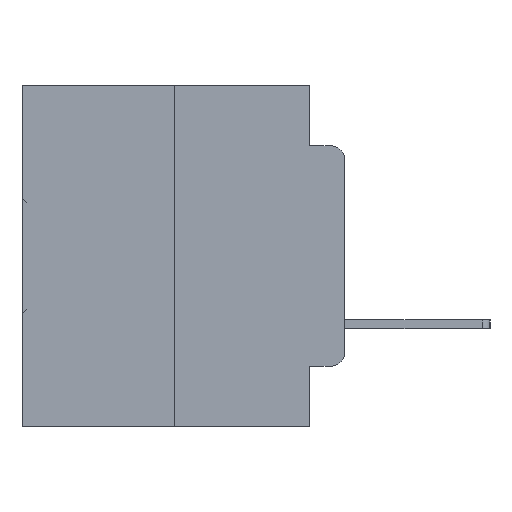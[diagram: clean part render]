
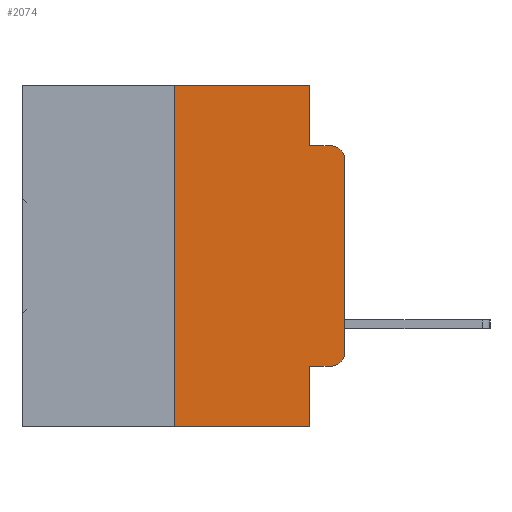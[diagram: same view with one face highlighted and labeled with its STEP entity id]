
A CAD part, left-side view. The second image highlights one B-rep face of the part: STEP entity #2074.
In plain terms, the highlighted planar face has unit normal (-1, 0, 0).
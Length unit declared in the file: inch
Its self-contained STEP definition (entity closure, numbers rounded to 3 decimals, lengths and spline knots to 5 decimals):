
#961 = EDGE_CURVE ( 'NONE', #13620, #11666, #12895, .T. ) ;
#1008 = VECTOR ( 'NONE', #7044, 39.37008 ) ;
#1554 = DIRECTION ( 'NONE',  ( 0., -1., 0. ) ) ;
#2074 = ADVANCED_FACE ( 'NONE', ( #23694 ), #25419, .F. ) ;
#2277 = ORIENTED_EDGE ( 'NONE', *, *, #2751, .T. ) ;
#2463 = ORIENTED_EDGE ( 'NONE', *, *, #961, .T. ) ;
#2751 = EDGE_CURVE ( 'NONE', #11666, #20165, #25672, .T. ) ;
#3891 = CARTESIAN_POINT ( 'NONE',  ( 0., 0.473, -0.5 ) ) ;
#4189 = ORIENTED_EDGE ( 'NONE', *, *, #15668, .F. ) ;
#5625 = LINE ( 'NONE', #25116, #13402 ) ;
#6487 = VERTEX_POINT ( 'NONE', #28314 ) ;
#6634 = LINE ( 'NONE', #17175, #19680 ) ;
#6671 = CARTESIAN_POINT ( 'NONE',  ( 0., 0.25, 0. ) ) ;
#6856 = EDGE_CURVE ( 'NONE', #26760, #13575, #19424, .T. ) ;
#7044 = DIRECTION ( 'NONE',  ( 0., 0., 1. ) ) ;
#7055 = DIRECTION ( 'NONE',  ( 0., 0., -1. ) ) ;
#7791 = ORIENTED_EDGE ( 'NONE', *, *, #6856, .T. ) ;
#8467 = CARTESIAN_POINT ( 'NONE',  ( 0., 0.051, -0.0885 ) ) ;
#8584 = ORIENTED_EDGE ( 'NONE', *, *, #30925, .F. ) ;
#8736 = AXIS2_PLACEMENT_3D ( 'NONE', #24629, #9180, #27189 ) ;
#8743 = LINE ( 'NONE', #14873, #1008 ) ;
#8964 = CARTESIAN_POINT ( 'NONE',  ( 0., 0.051, -0.4115 ) ) ;
#9180 = DIRECTION ( 'NONE',  ( -1., 0., 0. ) ) ;
#9181 = ORIENTED_EDGE ( 'NONE', *, *, #14524, .T. ) ;
#9754 = ORIENTED_EDGE ( 'NONE', *, *, #27592, .F. ) ;
#10502 = ORIENTED_EDGE ( 'NONE', *, *, #16811, .F. ) ;
#10653 = ORIENTED_EDGE ( 'NONE', *, *, #20800, .F. ) ;
#10763 = VERTEX_POINT ( 'NONE', #29283 ) ;
#11415 = CARTESIAN_POINT ( 'NONE',  ( 0., 0.25, -0.5 ) ) ;
#11505 = CARTESIAN_POINT ( 'NONE',  ( 0., 0.02, -0.0885 ) ) ;
#11506 = DIRECTION ( 'NONE',  ( 0., 0., 1. ) ) ;
#11666 = VERTEX_POINT ( 'NONE', #25038 ) ;
#11779 = VECTOR ( 'NONE', #1554, 39.37008 ) ;
#11822 = DIRECTION ( 'NONE',  ( 0., 0., -1. ) ) ;
#11830 = DIRECTION ( 'NONE',  ( -1., 0., 0. ) ) ;
#12587 = LINE ( 'NONE', #3891, #14226 ) ;
#12622 = LINE ( 'NONE', #32262, #11779 ) ;
#12838 = AXIS2_PLACEMENT_3D ( 'NONE', #14885, #11830, #11822 ) ;
#12895 = LINE ( 'NONE', #20677, #18947 ) ;
#13402 = VECTOR ( 'NONE', #7055, 39.37008 ) ;
#13575 = VERTEX_POINT ( 'NONE', #11505 ) ;
#13620 = VERTEX_POINT ( 'NONE', #8964 ) ;
#13757 = DIRECTION ( 'NONE',  ( 0., -1., 0. ) ) ;
#14226 = VECTOR ( 'NONE', #22008, 39.37008 ) ;
#14524 = EDGE_CURVE ( 'NONE', #24122, #10763, #12587, .T. ) ;
#14873 = CARTESIAN_POINT ( 'NONE',  ( 0., 0., 0. ) ) ;
#14885 = CARTESIAN_POINT ( 'NONE',  ( 0., 0.02, -0.3915 ) ) ;
#15668 = EDGE_CURVE ( 'NONE', #26739, #13575, #20224, .T. ) ;
#16811 = EDGE_CURVE ( 'NONE', #22449, #6487, #12622, .T. ) ;
#17175 = CARTESIAN_POINT ( 'NONE',  ( 0., 0.051, 0. ) ) ;
#18947 = VECTOR ( 'NONE', #24319, 39.37008 ) ;
#18984 = LINE ( 'NONE', #26858, #26516 ) ;
#19424 = CIRCLE ( 'NONE', #8736, 0.02 ) ;
#19680 = VECTOR ( 'NONE', #19743, 39.37008 ) ;
#19743 = DIRECTION ( 'NONE',  ( 0., 0., -1. ) ) ;
#19956 = AXIS2_PLACEMENT_3D ( 'NONE', #21521, #20945, #21151 ) ;
#20165 = VERTEX_POINT ( 'NONE', #23649 ) ;
#20224 = LINE ( 'NONE', #8467, #26146 ) ;
#20677 = CARTESIAN_POINT ( 'NONE',  ( 0., 0.051, -0.4115 ) ) ;
#20800 = EDGE_CURVE ( 'NONE', #6487, #26739, #5625, .T. ) ;
#20945 = DIRECTION ( 'NONE',  ( 1., 0., 0. ) ) ;
#21151 = DIRECTION ( 'NONE',  ( 0., 0., -1. ) ) ;
#21521 = CARTESIAN_POINT ( 'NONE',  ( 0., 0.473, 0. ) ) ;
#22008 = DIRECTION ( 'NONE',  ( 0., -1., 0. ) ) ;
#22449 = VERTEX_POINT ( 'NONE', #6671 ) ;
#23385 = CARTESIAN_POINT ( 'NONE',  ( 0., 0.051, -0.0885 ) ) ;
#23649 = CARTESIAN_POINT ( 'NONE',  ( 0., 0., -0.3915 ) ) ;
#23694 = FACE_OUTER_BOUND ( 'NONE', #29109, .T. ) ;
#24122 = VERTEX_POINT ( 'NONE', #11415 ) ;
#24319 = DIRECTION ( 'NONE',  ( 0., -1., 0. ) ) ;
#24629 = CARTESIAN_POINT ( 'NONE',  ( 0., 0.02, -0.1085 ) ) ;
#25038 = CARTESIAN_POINT ( 'NONE',  ( 0., 0.02, -0.4115 ) ) ;
#25116 = CARTESIAN_POINT ( 'NONE',  ( 0., 0.051, 0. ) ) ;
#25419 = PLANE ( 'NONE',  #19956 ) ;
#25672 = CIRCLE ( 'NONE', #12838, 0.02 ) ;
#26146 = VECTOR ( 'NONE', #13757, 39.37008 ) ;
#26516 = VECTOR ( 'NONE', #11506, 39.37008 ) ;
#26739 = VERTEX_POINT ( 'NONE', #23385 ) ;
#26760 = VERTEX_POINT ( 'NONE', #28579 ) ;
#26858 = CARTESIAN_POINT ( 'NONE',  ( 0., 0.25, 0. ) ) ;
#27189 = DIRECTION ( 'NONE',  ( 0., 0., -1. ) ) ;
#27592 = EDGE_CURVE ( 'NONE', #24122, #22449, #18984, .T. ) ;
#28218 = EDGE_CURVE ( 'NONE', #20165, #26760, #8743, .T. ) ;
#28314 = CARTESIAN_POINT ( 'NONE',  ( 0., 0.051, 0. ) ) ;
#28579 = CARTESIAN_POINT ( 'NONE',  ( 0., 0., -0.1085 ) ) ;
#29109 = EDGE_LOOP ( 'NONE', ( #31248, #7791, #4189, #10653, #10502, #9754, #9181, #8584, #2463, #2277 ) ) ;
#29283 = CARTESIAN_POINT ( 'NONE',  ( 0., 0.051, -0.5 ) ) ;
#30925 = EDGE_CURVE ( 'NONE', #13620, #10763, #6634, .T. ) ;
#31248 = ORIENTED_EDGE ( 'NONE', *, *, #28218, .T. ) ;
#32262 = CARTESIAN_POINT ( 'NONE',  ( 0., 0.473, 0. ) ) ;
